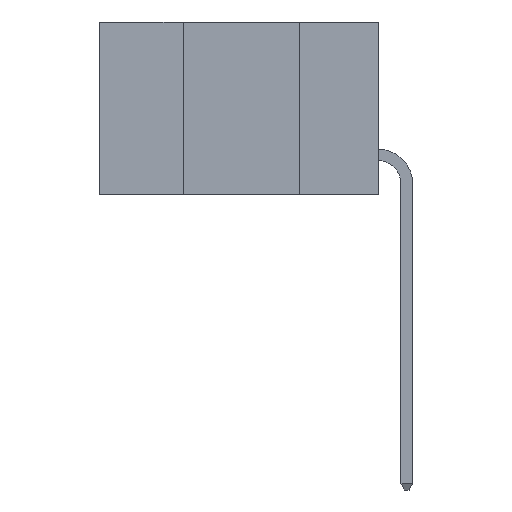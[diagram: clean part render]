
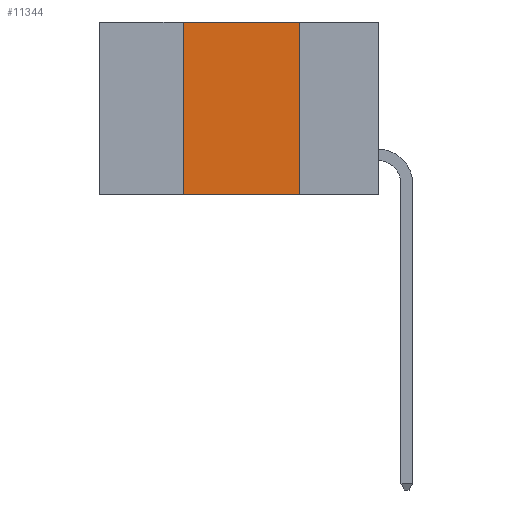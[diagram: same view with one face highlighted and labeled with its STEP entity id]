
A CAD part, left-side view. The second image highlights one B-rep face of the part: STEP entity #11344.
In plain terms, the highlighted planar face has unit normal (-1, 0, 0).
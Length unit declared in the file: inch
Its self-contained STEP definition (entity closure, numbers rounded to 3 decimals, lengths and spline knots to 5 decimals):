
#142 = CARTESIAN_POINT ( 'NONE',  ( 0., 0.17, 0. ) ) ;
#257 = CARTESIAN_POINT ( 'NONE',  ( 0., 0.42, -0.37 ) ) ;
#449 = VERTEX_POINT ( 'NONE', #571 ) ;
#501 = EDGE_CURVE ( 'NONE', #2801, #10235, #8602, .T. ) ;
#571 = CARTESIAN_POINT ( 'NONE',  ( 0., 0.42, 0. ) ) ;
#768 = ORIENTED_EDGE ( 'NONE', *, *, #2396, .T. ) ;
#779 = ORIENTED_EDGE ( 'NONE', *, *, #10321, .F. ) ;
#828 = ORIENTED_EDGE ( 'NONE', *, *, #1772, .F. ) ;
#1391 = EDGE_LOOP ( 'NONE', ( #5220, #828, #779, #768 ) ) ;
#1407 = VECTOR ( 'NONE', #8137, 39.37008 ) ;
#1428 = DIRECTION ( 'NONE',  ( 1., 0., 0. ) ) ;
#1772 = EDGE_CURVE ( 'NONE', #449, #2801, #9665, .T. ) ;
#2396 = EDGE_CURVE ( 'NONE', #9987, #10235, #5048, .T. ) ;
#2801 = VERTEX_POINT ( 'NONE', #142 ) ;
#4736 = FACE_OUTER_BOUND ( 'NONE', #1391, .T. ) ;
#4773 = VECTOR ( 'NONE', #5362, 39.37008 ) ;
#4900 = LINE ( 'NONE', #7207, #7046 ) ;
#5040 = PLANE ( 'NONE',  #6973 ) ;
#5048 = LINE ( 'NONE', #5435, #4773 ) ;
#5220 = ORIENTED_EDGE ( 'NONE', *, *, #501, .F. ) ;
#5362 = DIRECTION ( 'NONE',  ( 0., -1., 0. ) ) ;
#5435 = CARTESIAN_POINT ( 'NONE',  ( 0., 0.6, -0.37 ) ) ;
#6200 = CARTESIAN_POINT ( 'NONE',  ( 0., 0.17, -0.37 ) ) ;
#6896 = CARTESIAN_POINT ( 'NONE',  ( 0., 0.6, 0. ) ) ;
#6973 = AXIS2_PLACEMENT_3D ( 'NONE', #6896, #1428, #7757 ) ;
#7046 = VECTOR ( 'NONE', #7174, 39.37008 ) ;
#7070 = VECTOR ( 'NONE', #7217, 39.37008 ) ;
#7174 = DIRECTION ( 'NONE',  ( 0., 0., 1. ) ) ;
#7207 = CARTESIAN_POINT ( 'NONE',  ( 0., 0.42, -0.37 ) ) ;
#7217 = DIRECTION ( 'NONE',  ( 0., -1., 0. ) ) ;
#7280 = CARTESIAN_POINT ( 'NONE',  ( 0., 0.6, 0. ) ) ;
#7757 = DIRECTION ( 'NONE',  ( 0., 0., -1. ) ) ;
#8137 = DIRECTION ( 'NONE',  ( 0., 0., -1. ) ) ;
#8372 = CARTESIAN_POINT ( 'NONE',  ( 0., 0.17, -0.37 ) ) ;
#8602 = LINE ( 'NONE', #8372, #1407 ) ;
#9665 = LINE ( 'NONE', #7280, #7070 ) ;
#9987 = VERTEX_POINT ( 'NONE', #257 ) ;
#10235 = VERTEX_POINT ( 'NONE', #6200 ) ;
#10321 = EDGE_CURVE ( 'NONE', #9987, #449, #4900, .T. ) ;
#11344 = ADVANCED_FACE ( 'NONE', ( #4736 ), #5040, .F. ) ;
